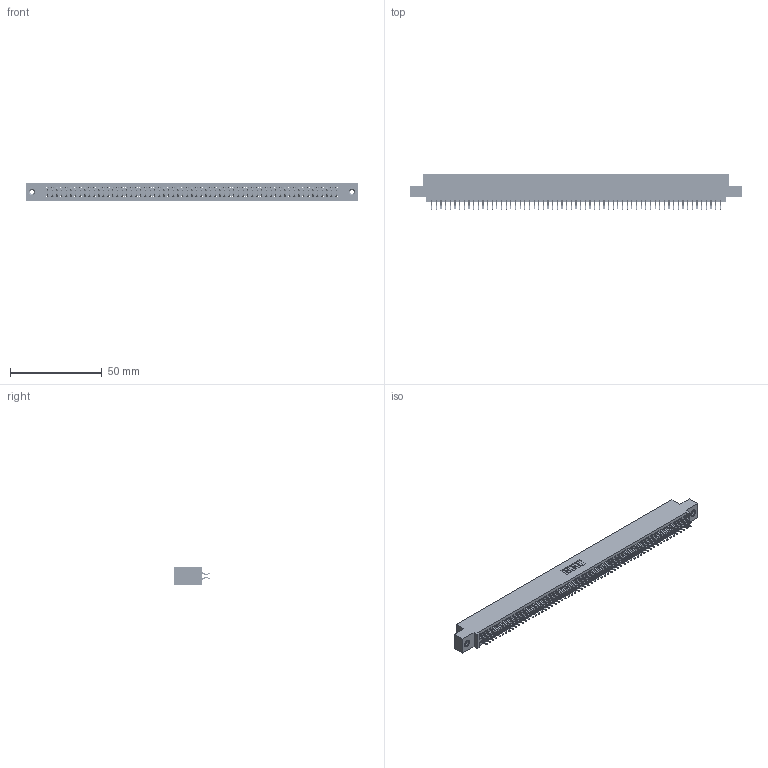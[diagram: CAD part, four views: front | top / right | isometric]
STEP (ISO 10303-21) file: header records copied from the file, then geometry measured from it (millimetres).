
FILE_DESCRIPTION (( 'STEP AP203' ), '1' );
FILE_NAME ('395-126-556-508.STEP', '2019-10-28T16:25:56', ( '' ), ( '' ), 'SwSTEP 2.0', 'SolidWorks 2016', '' );
FILE_SCHEMA (( 'CONFIG_CONTROL_DESIGN' ));
Length unit declared in the file: inch
Products named in the file (4): 345-250-001_345-250-003-102; 395-126-556-508; 345 Part_0.110 Offset - 0.156 Dia-TI; 345-292-001_556 Tail
Assembly tree (129 placements, depth 2):
  395-126-556-508
    345 Part_0.110 Offset - 0.156 Dia-TI
    345-292-001_556 Tail  x126
    345-250-001_345-250-003-102  x2
Bounding box: 181.23 x 19.24 x 9.4 mm (x, y, z)
Volume: 17714.8 mm3; surface area: 26588.2 mm2
Topology: 129 solids, 129 shells, 7246 faces, 21531 edges, 14178 vertices
Faces by surface type: plane 4778, cylinder 2452, cone 12, torus 4
Entity records: 48142 total; most frequent: CARTESIAN_POINT 8047, ORIENTED_EDGE 7962, DIRECTION 7083, EDGE_CURVE 3981, LINE 3569, VECTOR 3569, VERTEX_POINT 2648, AXIS2_PLACEMENT_3D 1757
